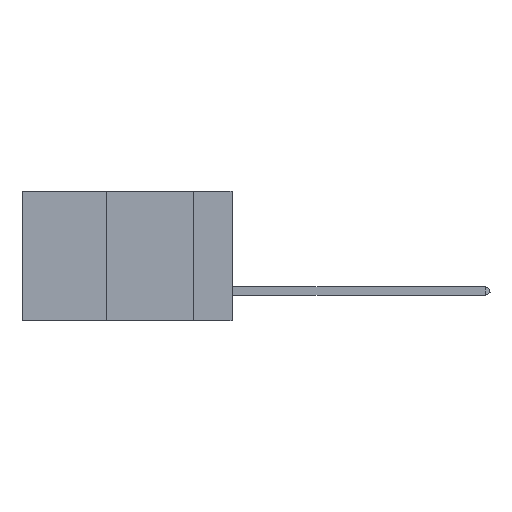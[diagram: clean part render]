
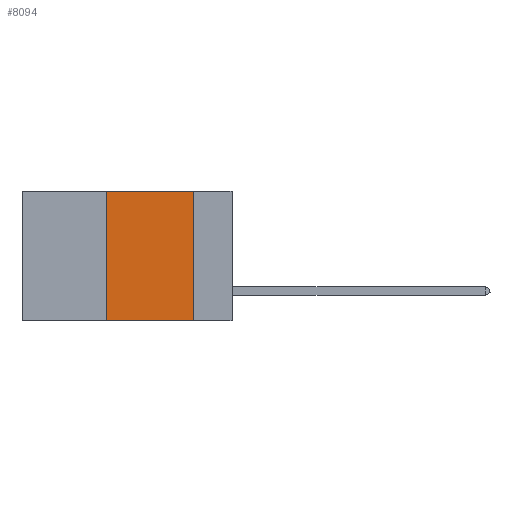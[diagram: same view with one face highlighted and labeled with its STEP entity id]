
A CAD part, left-side view. The second image highlights one B-rep face of the part: STEP entity #8094.
In plain terms, the highlighted planar face has unit normal (-1, 0, 0).
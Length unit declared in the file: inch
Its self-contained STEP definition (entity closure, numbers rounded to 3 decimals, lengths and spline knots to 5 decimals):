
#60 = ORIENTED_EDGE ( 'NONE', *, *, #15697, .F. ) ;
#417 = DIRECTION ( 'NONE',  ( 0., -1., 0. ) ) ;
#2559 = VERTEX_POINT ( 'NONE', #6222 ) ;
#4084 = DIRECTION ( 'NONE',  ( 0., -1., 0. ) ) ;
#6222 = CARTESIAN_POINT ( 'NONE',  ( 0., 0.36, 0. ) ) ;
#6299 = ORIENTED_EDGE ( 'NONE', *, *, #25847, .F. ) ;
#6405 = DIRECTION ( 'NONE',  ( 0., 0., -1. ) ) ;
#6432 = CARTESIAN_POINT ( 'NONE',  ( 0., 0.6, 0. ) ) ;
#6768 = CARTESIAN_POINT ( 'NONE',  ( 0., 0.11, 0. ) ) ;
#6813 = EDGE_LOOP ( 'NONE', ( #18840, #60, #6299, #20708 ) ) ;
#7600 = VERTEX_POINT ( 'NONE', #8738 ) ;
#8094 = ADVANCED_FACE ( 'NONE', ( #23125 ), #17871, .F. ) ;
#8738 = CARTESIAN_POINT ( 'NONE',  ( 0., 0.11, -0.37 ) ) ;
#9174 = DIRECTION ( 'NONE',  ( 1., 0., 0. ) ) ;
#10236 = VECTOR ( 'NONE', #21381, 39.37008 ) ;
#11882 = EDGE_CURVE ( 'NONE', #13719, #7600, #22945, .T. ) ;
#13497 = VERTEX_POINT ( 'NONE', #6768 ) ;
#13712 = LINE ( 'NONE', #6432, #18394 ) ;
#13719 = VERTEX_POINT ( 'NONE', #19634 ) ;
#15697 = EDGE_CURVE ( 'NONE', #2559, #13497, #13712, .T. ) ;
#16465 = CARTESIAN_POINT ( 'NONE',  ( 0., 0.11, 0. ) ) ;
#17268 = CARTESIAN_POINT ( 'NONE',  ( 0., 0.6, 0. ) ) ;
#17871 = PLANE ( 'NONE',  #18656 ) ;
#18394 = VECTOR ( 'NONE', #4084, 39.37008 ) ;
#18656 = AXIS2_PLACEMENT_3D ( 'NONE', #17268, #9174, #23402 ) ;
#18725 = LINE ( 'NONE', #19674, #10236 ) ;
#18840 = ORIENTED_EDGE ( 'NONE', *, *, #23497, .F. ) ;
#19634 = CARTESIAN_POINT ( 'NONE',  ( 0., 0.36, -0.37 ) ) ;
#19674 = CARTESIAN_POINT ( 'NONE',  ( 0., 0.36, 0. ) ) ;
#20708 = ORIENTED_EDGE ( 'NONE', *, *, #11882, .T. ) ;
#21381 = DIRECTION ( 'NONE',  ( 0., 0., 1. ) ) ;
#22945 = LINE ( 'NONE', #24850, #24203 ) ;
#23125 = FACE_OUTER_BOUND ( 'NONE', #6813, .T. ) ;
#23402 = DIRECTION ( 'NONE',  ( 0., 0., -1. ) ) ;
#23497 = EDGE_CURVE ( 'NONE', #13497, #7600, #24651, .T. ) ;
#24203 = VECTOR ( 'NONE', #417, 39.37008 ) ;
#24651 = LINE ( 'NONE', #16465, #25613 ) ;
#24850 = CARTESIAN_POINT ( 'NONE',  ( 0., 0.6, -0.37 ) ) ;
#25613 = VECTOR ( 'NONE', #6405, 39.37008 ) ;
#25847 = EDGE_CURVE ( 'NONE', #13719, #2559, #18725, .T. ) ;
